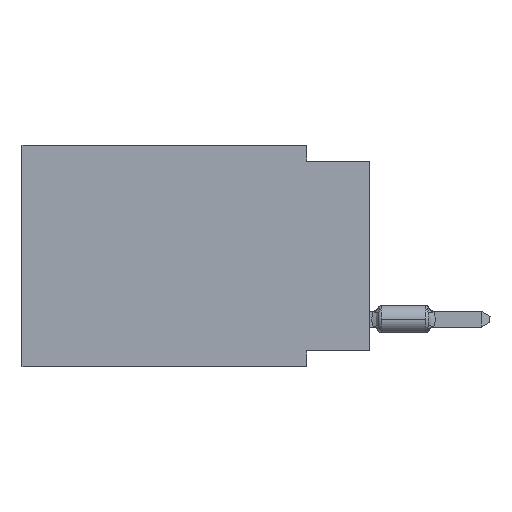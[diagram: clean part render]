
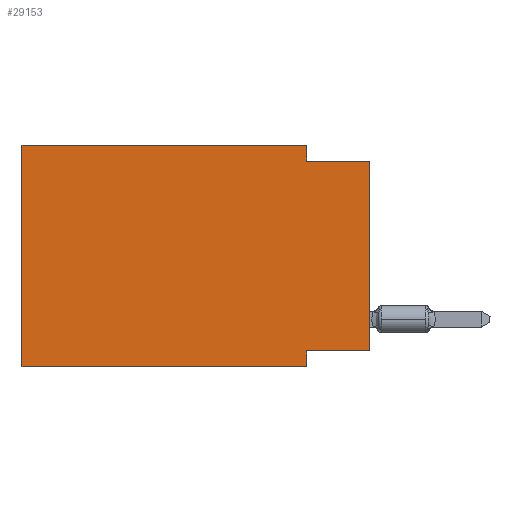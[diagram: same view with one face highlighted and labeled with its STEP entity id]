
A CAD part, left-side view. The second image highlights one B-rep face of the part: STEP entity #29153.
In plain terms, the highlighted planar face has unit normal (-1, 0, 0).
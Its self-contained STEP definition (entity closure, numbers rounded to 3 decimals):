
#294 = AXIS2_PLACEMENT_3D ( 'NONE', #30760, #50665, #50913 ) ;
#666 = ORIENTED_EDGE ( 'NONE', *, *, #1226, .F. ) ;
#786 = LINE ( 'NONE', #27965, #23426 ) ;
#1226 = EDGE_CURVE ( 'NONE', #27525, #28554, #786, .T. ) ;
#1724 = ORIENTED_EDGE ( 'NONE', *, *, #19879, .F. ) ;
#1807 = CARTESIAN_POINT ( 'NONE',  ( 0., 13.97, -8.89 ) ) ;
#1970 = EDGE_CURVE ( 'NONE', #37572, #37278, #25850, .T. ) ;
#2270 = CARTESIAN_POINT ( 'NONE',  ( 0., 0., -0.635 ) ) ;
#3869 = ORIENTED_EDGE ( 'NONE', *, *, #13949, .F. ) ;
#6060 = VECTOR ( 'NONE', #43388, 1000. ) ;
#6456 = LINE ( 'NONE', #26137, #13595 ) ;
#8332 = VERTEX_POINT ( 'NONE', #2270 ) ;
#9335 = CARTESIAN_POINT ( 'NONE',  ( 0., 0., -8.255 ) ) ;
#11337 = LINE ( 'NONE', #15469, #43559 ) ;
#12017 = ORIENTED_EDGE ( 'NONE', *, *, #24744, .T. ) ;
#12185 = DIRECTION ( 'NONE',  ( 0., 0., -1. ) ) ;
#13595 = VECTOR ( 'NONE', #30017, 1000. ) ;
#13596 = CARTESIAN_POINT ( 'NONE',  ( 0., 2.54, -8.255 ) ) ;
#13949 = EDGE_CURVE ( 'NONE', #20964, #33535, #29000, .T. ) ;
#14544 = CARTESIAN_POINT ( 'NONE',  ( 0., 2.54, -8.89 ) ) ;
#15469 = CARTESIAN_POINT ( 'NONE',  ( 0., 0., 0. ) ) ;
#17624 = DIRECTION ( 'NONE',  ( 0., 1., 0. ) ) ;
#18464 = LINE ( 'NONE', #24750, #25573 ) ;
#18850 = PLANE ( 'NONE',  #294 ) ;
#19409 = LINE ( 'NONE', #23554, #50627 ) ;
#19879 = EDGE_CURVE ( 'NONE', #33535, #37278, #18464, .T. ) ;
#20964 = VERTEX_POINT ( 'NONE', #27625 ) ;
#23036 = DIRECTION ( 'NONE',  ( 0., 0., 1. ) ) ;
#23321 = CARTESIAN_POINT ( 'NONE',  ( 0., 13.97, 0. ) ) ;
#23426 = VECTOR ( 'NONE', #12185, 1000. ) ;
#23554 = CARTESIAN_POINT ( 'NONE',  ( 0., 13.97, 0. ) ) ;
#24744 = EDGE_CURVE ( 'NONE', #20964, #8332, #11337, .T. ) ;
#24750 = CARTESIAN_POINT ( 'NONE',  ( 0., 2.54, -8.89 ) ) ;
#25432 = VECTOR ( 'NONE', #17624, 1000. ) ;
#25573 = VECTOR ( 'NONE', #32754, 1000. ) ;
#25850 = LINE ( 'NONE', #46251, #50709 ) ;
#26137 = CARTESIAN_POINT ( 'NONE',  ( 0., 0., -0.635 ) ) ;
#27145 = EDGE_LOOP ( 'NONE', ( #12017, #45286, #666, #37295, #38926, #39551, #1724, #3869 ) ) ;
#27525 = VERTEX_POINT ( 'NONE', #28638 ) ;
#27625 = CARTESIAN_POINT ( 'NONE',  ( 0., 0., -8.255 ) ) ;
#27965 = CARTESIAN_POINT ( 'NONE',  ( 0., 2.54, 0. ) ) ;
#28382 = LINE ( 'NONE', #31492, #6060 ) ;
#28554 = VERTEX_POINT ( 'NONE', #33672 ) ;
#28638 = CARTESIAN_POINT ( 'NONE',  ( 0., 2.54, 0. ) ) ;
#29000 = LINE ( 'NONE', #9335, #25432 ) ;
#29153 = ADVANCED_FACE ( 'NONE', ( #34642 ), #18850, .F. ) ;
#30017 = DIRECTION ( 'NONE',  ( 0., -1., 0. ) ) ;
#30760 = CARTESIAN_POINT ( 'NONE',  ( 0., 13.97, 0. ) ) ;
#31264 = VERTEX_POINT ( 'NONE', #23321 ) ;
#31492 = CARTESIAN_POINT ( 'NONE',  ( 0., 13.97, 0. ) ) ;
#31532 = EDGE_CURVE ( 'NONE', #28554, #8332, #6456, .T. ) ;
#32754 = DIRECTION ( 'NONE',  ( 0., 0., -1. ) ) ;
#33535 = VERTEX_POINT ( 'NONE', #13596 ) ;
#33672 = CARTESIAN_POINT ( 'NONE',  ( 0., 2.54, -0.635 ) ) ;
#34642 = FACE_OUTER_BOUND ( 'NONE', #27145, .T. ) ;
#37278 = VERTEX_POINT ( 'NONE', #14544 ) ;
#37295 = ORIENTED_EDGE ( 'NONE', *, *, #41912, .F. ) ;
#37572 = VERTEX_POINT ( 'NONE', #1807 ) ;
#37733 = DIRECTION ( 'NONE',  ( 0., -1., 0. ) ) ;
#38926 = ORIENTED_EDGE ( 'NONE', *, *, #41326, .F. ) ;
#39551 = ORIENTED_EDGE ( 'NONE', *, *, #1970, .T. ) ;
#41326 = EDGE_CURVE ( 'NONE', #37572, #31264, #19409, .T. ) ;
#41912 = EDGE_CURVE ( 'NONE', #31264, #27525, #28382, .T. ) ;
#42874 = DIRECTION ( 'NONE',  ( 0., 0., 1. ) ) ;
#43388 = DIRECTION ( 'NONE',  ( 0., -1., 0. ) ) ;
#43559 = VECTOR ( 'NONE', #42874, 1000. ) ;
#45286 = ORIENTED_EDGE ( 'NONE', *, *, #31532, .F. ) ;
#46251 = CARTESIAN_POINT ( 'NONE',  ( 0., 13.97, -8.89 ) ) ;
#50627 = VECTOR ( 'NONE', #23036, 1000. ) ;
#50665 = DIRECTION ( 'NONE',  ( 1., 0., 0. ) ) ;
#50709 = VECTOR ( 'NONE', #37733, 1000. ) ;
#50913 = DIRECTION ( 'NONE',  ( 0., 0., -1. ) ) ;
